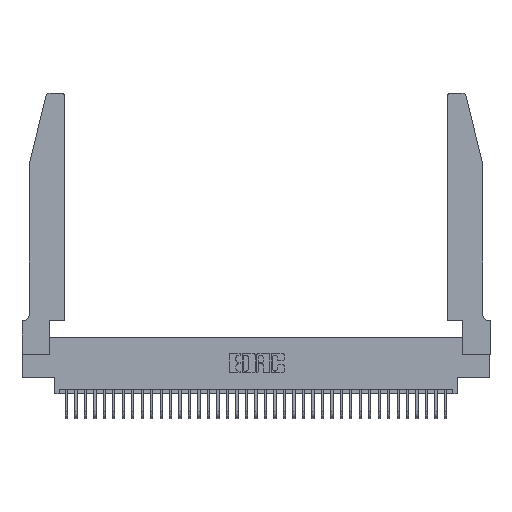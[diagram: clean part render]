
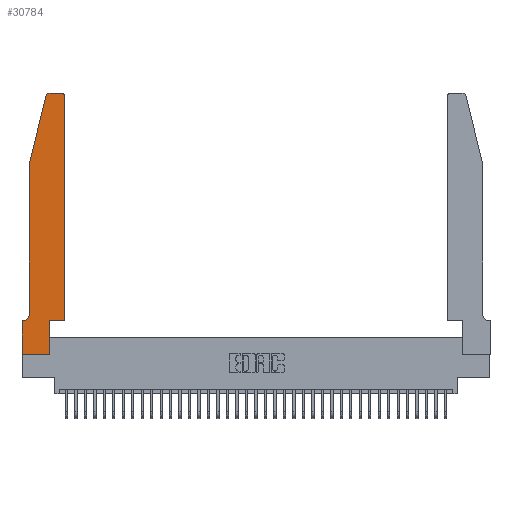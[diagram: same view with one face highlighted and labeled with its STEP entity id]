
A CAD part, top view. The second image highlights one B-rep face of the part: STEP entity #30784.
In plain terms, the highlighted planar face has unit normal (0, 0, 1).
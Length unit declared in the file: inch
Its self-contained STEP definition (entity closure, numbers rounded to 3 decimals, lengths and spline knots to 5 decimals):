
#298 = VECTOR ( 'NONE', #30539, 39.37008 ) ;
#435 = LINE ( 'NONE', #13225, #20861 ) ;
#1423 = EDGE_CURVE ( 'NONE', #35255, #17517, #13623, .T. ) ;
#1470 = DIRECTION ( 'NONE',  ( -1., 0., 0. ) ) ;
#1601 = CARTESIAN_POINT ( 'NONE',  ( 0.2605, 2.75, 0.37 ) ) ;
#1797 = EDGE_CURVE ( 'NONE', #10041, #23528, #15321, .T. ) ;
#2489 = EDGE_LOOP ( 'NONE', ( #14491, #4148, #7930, #13368, #12659, #25081, #3617, #23685, #22378, #33657, #14799, #32535 ) ) ;
#3617 = ORIENTED_EDGE ( 'NONE', *, *, #16671, .T. ) ;
#3702 = CIRCLE ( 'NONE', #17819, 0.07 ) ;
#4084 = CARTESIAN_POINT ( 'NONE',  ( 0., 0., 0.37 ) ) ;
#4148 = ORIENTED_EDGE ( 'NONE', *, *, #4830, .T. ) ;
#4208 = DIRECTION ( 'NONE',  ( 1., 0., 0. ) ) ;
#4530 = DIRECTION ( 'NONE',  ( 0., 0., 1. ) ) ;
#4830 = EDGE_CURVE ( 'NONE', #31102, #20948, #23335, .T. ) ;
#4852 = CARTESIAN_POINT ( 'NONE',  ( 0.0755, 2., 0.37 ) ) ;
#5424 = CARTESIAN_POINT ( 'NONE',  ( 0., 0., 0.37 ) ) ;
#5680 = CARTESIAN_POINT ( 'NONE',  ( 0.0755, 2., 0.37 ) ) ;
#6137 = CARTESIAN_POINT ( 'NONE',  ( 0., 0.35, 0.37 ) ) ;
#6148 = CIRCLE ( 'NONE', #34698, 0.03 ) ;
#6265 = EDGE_CURVE ( 'NONE', #20948, #10041, #9758, .T. ) ;
#6486 = EDGE_CURVE ( 'NONE', #17517, #8793, #14914, .T. ) ;
#7565 = VECTOR ( 'NONE', #20171, 39.37008 ) ;
#7930 = ORIENTED_EDGE ( 'NONE', *, *, #6265, .T. ) ;
#7963 = VECTOR ( 'NONE', #8481, 39.37008 ) ;
#8195 = CARTESIAN_POINT ( 'NONE',  ( 0.4205, 2.75, 0.37 ) ) ;
#8380 = CARTESIAN_POINT ( 'NONE',  ( 0.4505, 0.35, 0.37 ) ) ;
#8481 = DIRECTION ( 'NONE',  ( 0., -1., 0. ) ) ;
#8517 = CARTESIAN_POINT ( 'NONE',  ( 0.25487, 2.72718, 0.37 ) ) ;
#8603 = EDGE_CURVE ( 'NONE', #35588, #14308, #435, .T. ) ;
#8666 = DIRECTION ( 'NONE',  ( 0., -1., 0. ) ) ;
#8793 = VERTEX_POINT ( 'NONE', #12687 ) ;
#9758 = LINE ( 'NONE', #27317, #21914 ) ;
#9947 = LINE ( 'NONE', #28031, #32037 ) ;
#10041 = VERTEX_POINT ( 'NONE', #4852 ) ;
#10127 = EDGE_CURVE ( 'NONE', #8793, #14905, #28945, .T. ) ;
#10978 = EDGE_CURVE ( 'NONE', #23528, #35588, #3702, .T. ) ;
#12117 = VECTOR ( 'NONE', #18248, 39.37008 ) ;
#12140 = CARTESIAN_POINT ( 'NONE',  ( 0.284, 2.72, 0.37 ) ) ;
#12196 = AXIS2_PLACEMENT_3D ( 'NONE', #29397, #4530, #23961 ) ;
#12659 = ORIENTED_EDGE ( 'NONE', *, *, #10978, .T. ) ;
#12687 = CARTESIAN_POINT ( 'NONE',  ( 0.2865, 0.35, 0.37 ) ) ;
#13225 = CARTESIAN_POINT ( 'NONE',  ( 0.0755, 0.35, 0.37 ) ) ;
#13368 = ORIENTED_EDGE ( 'NONE', *, *, #1797, .T. ) ;
#13623 = LINE ( 'NONE', #4084, #20136 ) ;
#14308 = VERTEX_POINT ( 'NONE', #6137 ) ;
#14491 = ORIENTED_EDGE ( 'NONE', *, *, #16401, .T. ) ;
#14799 = ORIENTED_EDGE ( 'NONE', *, *, #26983, .T. ) ;
#14905 = VERTEX_POINT ( 'NONE', #22721 ) ;
#14914 = LINE ( 'NONE', #17364, #7565 ) ;
#14917 = DIRECTION ( 'NONE',  ( 1., 0., 0. ) ) ;
#15076 = LINE ( 'NONE', #30734, #28950 ) ;
#15321 = LINE ( 'NONE', #5680, #7963 ) ;
#16362 = CARTESIAN_POINT ( 'NONE',  ( 0.4205, 2.72, 0.37 ) ) ;
#16401 = EDGE_CURVE ( 'NONE', #20252, #31102, #34221, .T. ) ;
#16671 = EDGE_CURVE ( 'NONE', #14308, #35255, #9947, .T. ) ;
#16785 = VERTEX_POINT ( 'NONE', #20043 ) ;
#17364 = CARTESIAN_POINT ( 'NONE',  ( 0.2865, 0.35, 0.37 ) ) ;
#17517 = VERTEX_POINT ( 'NONE', #20458 ) ;
#17819 = AXIS2_PLACEMENT_3D ( 'NONE', #34703, #18114, #1470 ) ;
#18114 = DIRECTION ( 'NONE',  ( 0., 0., -1. ) ) ;
#18248 = DIRECTION ( 'NONE',  ( -1., 0., 0. ) ) ;
#18375 = PLANE ( 'NONE',  #12196 ) ;
#18449 = EDGE_CURVE ( 'NONE', #16785, #20252, #6148, .T. ) ;
#19175 = DIRECTION ( 'NONE',  ( 1., 0., 0. ) ) ;
#20043 = CARTESIAN_POINT ( 'NONE',  ( 0.4505, 2.72, 0.37 ) ) ;
#20136 = VECTOR ( 'NONE', #4208, 39.37008 ) ;
#20171 = DIRECTION ( 'NONE',  ( 0., 1., 0. ) ) ;
#20252 = VERTEX_POINT ( 'NONE', #8195 ) ;
#20458 = CARTESIAN_POINT ( 'NONE',  ( 0.2865, 0., 0.37 ) ) ;
#20861 = VECTOR ( 'NONE', #21618, 39.37008 ) ;
#20948 = VERTEX_POINT ( 'NONE', #8517 ) ;
#21618 = DIRECTION ( 'NONE',  ( -1., 0., 0. ) ) ;
#21914 = VECTOR ( 'NONE', #24673, 39.37008 ) ;
#22378 = ORIENTED_EDGE ( 'NONE', *, *, #6486, .T. ) ;
#22623 = CARTESIAN_POINT ( 'NONE',  ( 0.284, 2.75, 0.37 ) ) ;
#22721 = CARTESIAN_POINT ( 'NONE',  ( 0.4505, 0.35, 0.37 ) ) ;
#23053 = CARTESIAN_POINT ( 'NONE',  ( 0.0755, 0.42, 0.37 ) ) ;
#23335 = CIRCLE ( 'NONE', #34999, 0.03 ) ;
#23474 = CARTESIAN_POINT ( 'NONE',  ( 0.0055, 0.35, 0.37 ) ) ;
#23528 = VERTEX_POINT ( 'NONE', #23053 ) ;
#23685 = ORIENTED_EDGE ( 'NONE', *, *, #1423, .T. ) ;
#23961 = DIRECTION ( 'NONE',  ( 1., 0., 0. ) ) ;
#24673 = DIRECTION ( 'NONE',  ( -0.239, -0.971, 0. ) ) ;
#25081 = ORIENTED_EDGE ( 'NONE', *, *, #8603, .T. ) ;
#26238 = FACE_OUTER_BOUND ( 'NONE', #2489, .T. ) ;
#26983 = EDGE_CURVE ( 'NONE', #14905, #16785, #15076, .T. ) ;
#27317 = CARTESIAN_POINT ( 'NONE',  ( 0.0755, 2., 0.37 ) ) ;
#28031 = CARTESIAN_POINT ( 'NONE',  ( 0., 0., 0.37 ) ) ;
#28945 = LINE ( 'NONE', #8380, #298 ) ;
#28950 = VECTOR ( 'NONE', #33510, 39.37008 ) ;
#29397 = CARTESIAN_POINT ( 'NONE',  ( 0., 0.35, 0.37 ) ) ;
#30539 = DIRECTION ( 'NONE',  ( 1., 0., 0. ) ) ;
#30734 = CARTESIAN_POINT ( 'NONE',  ( 0.4505, 0.35, 0.37 ) ) ;
#30784 = ADVANCED_FACE ( 'NONE', ( #26238 ), #18375, .T. ) ;
#31102 = VERTEX_POINT ( 'NONE', #22623 ) ;
#31522 = DIRECTION ( 'NONE',  ( 0., 0., 1. ) ) ;
#32037 = VECTOR ( 'NONE', #8666, 39.37008 ) ;
#32535 = ORIENTED_EDGE ( 'NONE', *, *, #18449, .T. ) ;
#33510 = DIRECTION ( 'NONE',  ( 0., 1., 0. ) ) ;
#33657 = ORIENTED_EDGE ( 'NONE', *, *, #10127, .T. ) ;
#34221 = LINE ( 'NONE', #1601, #12117 ) ;
#34698 = AXIS2_PLACEMENT_3D ( 'NONE', #16362, #35771, #19175 ) ;
#34703 = CARTESIAN_POINT ( 'NONE',  ( 0.0055, 0.42, 0.37 ) ) ;
#34999 = AXIS2_PLACEMENT_3D ( 'NONE', #12140, #31522, #14917 ) ;
#35255 = VERTEX_POINT ( 'NONE', #5424 ) ;
#35588 = VERTEX_POINT ( 'NONE', #23474 ) ;
#35771 = DIRECTION ( 'NONE',  ( 0., 0., 1. ) ) ;
